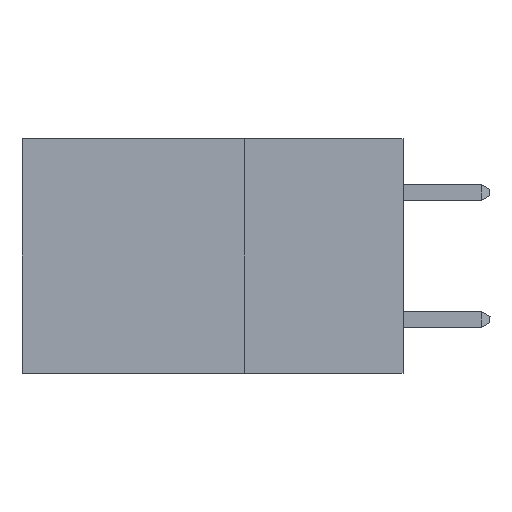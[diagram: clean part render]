
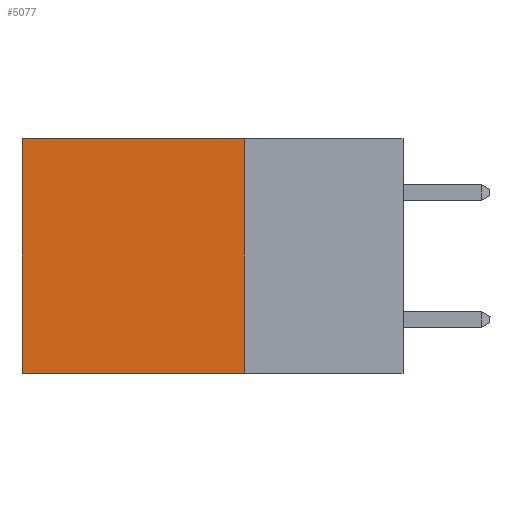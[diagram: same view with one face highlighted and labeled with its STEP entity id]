
A CAD part, left-side view. The second image highlights one B-rep face of the part: STEP entity #5077.
In plain terms, the highlighted planar face has unit normal (-1, 0, 0).
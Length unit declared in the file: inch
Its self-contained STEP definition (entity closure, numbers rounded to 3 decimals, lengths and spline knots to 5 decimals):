
#156 = ORIENTED_EDGE ( 'NONE', *, *, #5769, .T. ) ;
#517 = EDGE_LOOP ( 'NONE', ( #156, #2709, #17676, #17504 ) ) ;
#647 = CARTESIAN_POINT ( 'NONE',  ( 0.2875, 0.6, -0.37 ) ) ;
#2709 = ORIENTED_EDGE ( 'NONE', *, *, #19657, .F. ) ;
#3519 = EDGE_CURVE ( 'NONE', #5515, #20907, #16927, .T. ) ;
#4069 = LINE ( 'NONE', #21456, #11596 ) ;
#4997 = AXIS2_PLACEMENT_3D ( 'NONE', #21392, #5322, #7170 ) ;
#5070 = DIRECTION ( 'NONE',  ( 0., 1., 0. ) ) ;
#5077 = ADVANCED_FACE ( 'NONE', ( #10253 ), #5398, .F. ) ;
#5322 = DIRECTION ( 'NONE',  ( 1., 0., 0. ) ) ;
#5398 = PLANE ( 'NONE',  #4997 ) ;
#5515 = VERTEX_POINT ( 'NONE', #7896 ) ;
#5769 = EDGE_CURVE ( 'NONE', #20907, #18706, #4069, .T. ) ;
#6871 = VECTOR ( 'NONE', #5070, 39.37008 ) ;
#6893 = LINE ( 'NONE', #8318, #19225 ) ;
#7125 = VERTEX_POINT ( 'NONE', #11539 ) ;
#7170 = DIRECTION ( 'NONE',  ( 0., 0., -1. ) ) ;
#7896 = CARTESIAN_POINT ( 'NONE',  ( 0.2875, 0.25, 0. ) ) ;
#8318 = CARTESIAN_POINT ( 'NONE',  ( 0.2875, 0.25, -0.37 ) ) ;
#10176 = CARTESIAN_POINT ( 'NONE',  ( 0.2875, 0.6, 0. ) ) ;
#10253 = FACE_OUTER_BOUND ( 'NONE', #517, .T. ) ;
#10943 = CARTESIAN_POINT ( 'NONE',  ( 0.2875, 0.25, 0. ) ) ;
#11539 = CARTESIAN_POINT ( 'NONE',  ( 0.2875, 0.25, -0.37 ) ) ;
#11596 = VECTOR ( 'NONE', #14348, 39.37008 ) ;
#12474 = VECTOR ( 'NONE', #16433, 39.37008 ) ;
#14051 = DIRECTION ( 'NONE',  ( 0., 1., 0. ) ) ;
#14348 = DIRECTION ( 'NONE',  ( 0., 0., -1. ) ) ;
#15578 = EDGE_CURVE ( 'NONE', #5515, #7125, #21209, .T. ) ;
#16433 = DIRECTION ( 'NONE',  ( 0., 0., -1. ) ) ;
#16927 = LINE ( 'NONE', #22762, #6871 ) ;
#17504 = ORIENTED_EDGE ( 'NONE', *, *, #3519, .T. ) ;
#17676 = ORIENTED_EDGE ( 'NONE', *, *, #15578, .F. ) ;
#18706 = VERTEX_POINT ( 'NONE', #647 ) ;
#19225 = VECTOR ( 'NONE', #14051, 39.37008 ) ;
#19657 = EDGE_CURVE ( 'NONE', #7125, #18706, #6893, .T. ) ;
#20907 = VERTEX_POINT ( 'NONE', #10176 ) ;
#21209 = LINE ( 'NONE', #10943, #12474 ) ;
#21392 = CARTESIAN_POINT ( 'NONE',  ( 0.2875, 0.25, 0. ) ) ;
#21456 = CARTESIAN_POINT ( 'NONE',  ( 0.2875, 0.6, 0. ) ) ;
#22762 = CARTESIAN_POINT ( 'NONE',  ( 0.2875, 0.25, 0. ) ) ;
